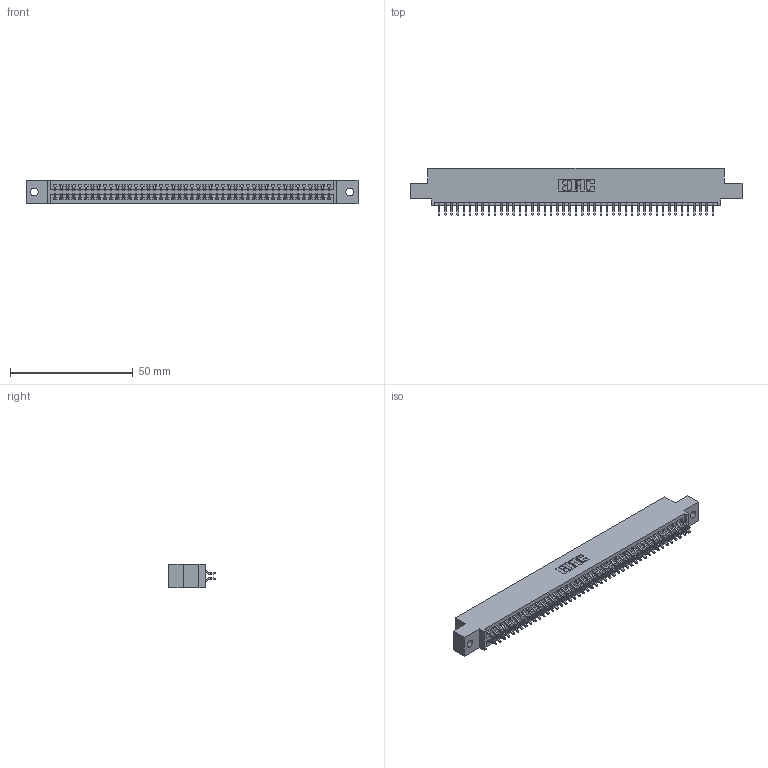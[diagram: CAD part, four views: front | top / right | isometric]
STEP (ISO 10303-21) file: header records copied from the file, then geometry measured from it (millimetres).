
FILE_DESCRIPTION (( 'STEP AP203' ), '1' );
FILE_NAME ('345-090-556-502.STEP', '2019-11-01T16:56:46', ( '' ), ( '' ), 'SwSTEP 2.0', 'SolidWorks 2016', '' );
FILE_SCHEMA (( 'CONFIG_CONTROL_DESIGN' ));
Length unit declared in the file: inch
Products named in the file (3): 345 Part_0.110 Offset - 0.128 Dia; 345-090-556-502; 345-292-001_556 Tail
Assembly tree (91 placements, depth 2):
  345-090-556-502
    345 Part_0.110 Offset - 0.128 Dia
    345-292-001_556 Tail  x90
Bounding box: 135.51 x 19.24 x 9.4 mm (x, y, z)
Volume: 13077.7 mm3; surface area: 19130.5 mm2
Topology: 91 solids, 91 shells, 5170 faces, 15383 edges, 10134 vertices
Faces by surface type: plane 3414, cylinder 1756
Entity records: 35259 total; most frequent: CARTESIAN_POINT 5924, ORIENTED_EDGE 5846, DIRECTION 5207, EDGE_CURVE 2923, LINE 2603, VECTOR 2603, VERTEX_POINT 1946, AXIS2_PLACEMENT_3D 1302
